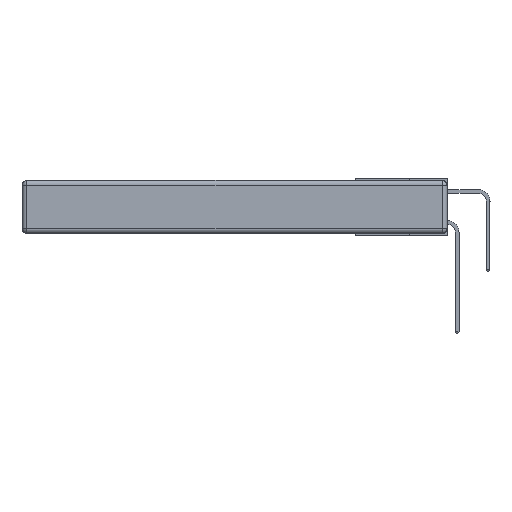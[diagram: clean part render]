
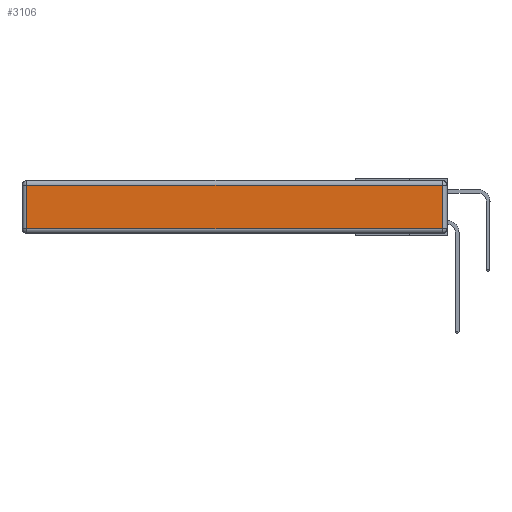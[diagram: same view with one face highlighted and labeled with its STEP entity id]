
A CAD part, left-side view. The second image highlights one B-rep face of the part: STEP entity #3106.
In plain terms, the highlighted planar face has unit normal (-1, 0, 0).
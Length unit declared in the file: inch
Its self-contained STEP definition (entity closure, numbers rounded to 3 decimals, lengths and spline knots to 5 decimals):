
#745 = CARTESIAN_POINT ( 'NONE',  ( 0., 2.72, -0.313 ) ) ;
#1036 = EDGE_CURVE ( 'NONE', #13890, #14619, #15285, .T. ) ;
#2482 = LINE ( 'NONE', #3297, #3036 ) ;
#2568 = ORIENTED_EDGE ( 'NONE', *, *, #17961, .T. ) ;
#2815 = LINE ( 'NONE', #13352, #20142 ) ;
#3036 = VECTOR ( 'NONE', #7825, 39.37008 ) ;
#3106 = ADVANCED_FACE ( 'NONE', ( #19863 ), #15420, .T. ) ;
#3297 = CARTESIAN_POINT ( 'NONE',  ( 0., 2.72, -0.343 ) ) ;
#3619 = EDGE_CURVE ( 'NONE', #12331, #22059, #2482, .T. ) ;
#3929 = CARTESIAN_POINT ( 'NONE',  ( 0., 0.03, -0.03 ) ) ;
#4372 = DIRECTION ( 'NONE',  ( 0., 0., 1. ) ) ;
#4489 = DIRECTION ( 'NONE',  ( 0., 1., 0. ) ) ;
#5604 = ORIENTED_EDGE ( 'NONE', *, *, #1036, .T. ) ;
#5962 = CARTESIAN_POINT ( 'NONE',  ( 0., 0.03, -0.343 ) ) ;
#6174 = VECTOR ( 'NONE', #13289, 39.37008 ) ;
#7821 = EDGE_LOOP ( 'NONE', ( #9192, #5604, #2568, #10108 ) ) ;
#7825 = DIRECTION ( 'NONE',  ( 0., 0., -1. ) ) ;
#8469 = LINE ( 'NONE', #20125, #13866 ) ;
#9192 = ORIENTED_EDGE ( 'NONE', *, *, #12804, .T. ) ;
#10108 = ORIENTED_EDGE ( 'NONE', *, *, #3619, .T. ) ;
#10883 = DIRECTION ( 'NONE',  ( 0., -1., 0. ) ) ;
#12331 = VERTEX_POINT ( 'NONE', #16390 ) ;
#12717 = CARTESIAN_POINT ( 'NONE',  ( 0., 0.03, -0.313 ) ) ;
#12804 = EDGE_CURVE ( 'NONE', #22059, #13890, #8469, .T. ) ;
#13289 = DIRECTION ( 'NONE',  ( 0., 0., 1. ) ) ;
#13352 = CARTESIAN_POINT ( 'NONE',  ( 0., 2.75, -0.03 ) ) ;
#13866 = VECTOR ( 'NONE', #10883, 39.37008 ) ;
#13890 = VERTEX_POINT ( 'NONE', #12717 ) ;
#14619 = VERTEX_POINT ( 'NONE', #3929 ) ;
#15285 = LINE ( 'NONE', #5962, #6174 ) ;
#15299 = AXIS2_PLACEMENT_3D ( 'NONE', #22559, #19044, #4372 ) ;
#15420 = PLANE ( 'NONE',  #15299 ) ;
#16390 = CARTESIAN_POINT ( 'NONE',  ( 0., 2.72, -0.03 ) ) ;
#17961 = EDGE_CURVE ( 'NONE', #14619, #12331, #2815, .T. ) ;
#19044 = DIRECTION ( 'NONE',  ( -1., 0., 0. ) ) ;
#19863 = FACE_OUTER_BOUND ( 'NONE', #7821, .T. ) ;
#20125 = CARTESIAN_POINT ( 'NONE',  ( 0., 0., -0.313 ) ) ;
#20142 = VECTOR ( 'NONE', #4489, 39.37008 ) ;
#22059 = VERTEX_POINT ( 'NONE', #745 ) ;
#22559 = CARTESIAN_POINT ( 'NONE',  ( 0., 0., -0.343 ) ) ;
